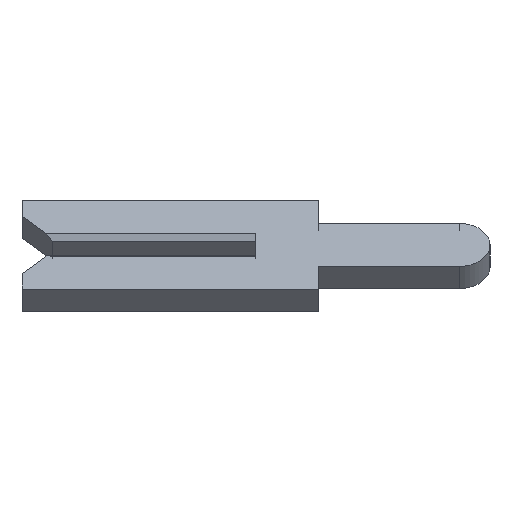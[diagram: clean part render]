
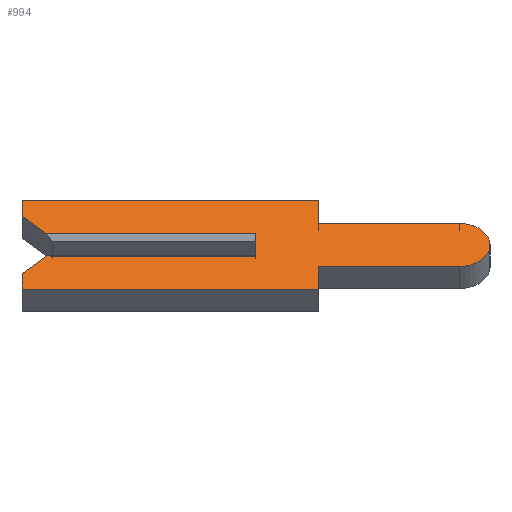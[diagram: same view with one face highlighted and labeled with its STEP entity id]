
A CAD part, left-side view. The second image highlights one B-rep face of the part: STEP entity #994.
In plain terms, the highlighted face is planar.
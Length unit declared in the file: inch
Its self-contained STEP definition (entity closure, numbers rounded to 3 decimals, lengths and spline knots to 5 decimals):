
#24 = VECTOR ( 'NONE', #486, 39.37008 ) ;
#33 = CARTESIAN_POINT ( 'NONE',  ( -0.01, -0.04, -0.04 ) ) ;
#35 = VERTEX_POINT ( 'NONE', #1326 ) ;
#36 = CARTESIAN_POINT ( 'NONE',  ( -0.01, 0.1305, -0.0065 ) ) ;
#39 = DIRECTION ( 'NONE',  ( 0., -0.707, 0.707 ) ) ;
#102 = EDGE_CURVE ( 'NONE', #569, #1413, #1185, .T. ) ;
#128 = CARTESIAN_POINT ( 'NONE',  ( -0.01, -0.04, 0.0195 ) ) ;
#132 = CARTESIAN_POINT ( 'NONE',  ( -0.01, 0.15, -0.04 ) ) ;
#154 = DIRECTION ( 'NONE',  ( 0., 0.707, 0.707 ) ) ;
#156 = EDGE_CURVE ( 'NONE', #281, #1231, #1251, .T. ) ;
#157 = VERTEX_POINT ( 'NONE', #472 ) ;
#158 = CARTESIAN_POINT ( 'NONE',  ( -0.01, 0.15, 0.04 ) ) ;
#165 = LINE ( 'NONE', #128, #1533 ) ;
#169 = LINE ( 'NONE', #1474, #1319 ) ;
#188 = DIRECTION ( 'NONE',  ( 0., -1., 0. ) ) ;
#198 = PLANE ( 'NONE',  #1428 ) ;
#204 = VECTOR ( 'NONE', #347, 39.37008 ) ;
#212 = ORIENTED_EDGE ( 'NONE', *, *, #927, .T. ) ;
#229 = CARTESIAN_POINT ( 'NONE',  ( -0.01, 0., 0.0065 ) ) ;
#237 = LINE ( 'NONE', #675, #1162 ) ;
#255 = EDGE_CURVE ( 'NONE', #788, #157, #1330, .T. ) ;
#275 = DIRECTION ( 'NONE',  ( 0., 0., -1. ) ) ;
#281 = VERTEX_POINT ( 'NONE', #132 ) ;
#306 = CARTESIAN_POINT ( 'NONE',  ( -0.01, -0.04, 0.04 ) ) ;
#311 = DIRECTION ( 'NONE',  ( 0., 0., -1. ) ) ;
#315 = ORIENTED_EDGE ( 'NONE', *, *, #1003, .F. ) ;
#321 = DIRECTION ( 'NONE',  ( 1., 0., 0. ) ) ;
#339 = EDGE_CURVE ( 'NONE', #1231, #1271, #1350, .T. ) ;
#347 = DIRECTION ( 'NONE',  ( 0., 0., 1. ) ) ;
#354 = VECTOR ( 'NONE', #188, 39.37008 ) ;
#362 = ORIENTED_EDGE ( 'NONE', *, *, #102, .F. ) ;
#424 = EDGE_CURVE ( 'NONE', #673, #788, #1155, .T. ) ;
#437 = EDGE_LOOP ( 'NONE', ( #212, #362, #588, #690, #961, #549, #1166, #315, #937, #693, #1250, #1091, #747, #1484 ) ) ;
#443 = VERTEX_POINT ( 'NONE', #644 ) ;
#448 = VECTOR ( 'NONE', #963, 39.37008 ) ;
#472 = CARTESIAN_POINT ( 'NONE',  ( -0.01, -0.04, 0.0195 ) ) ;
#486 = DIRECTION ( 'NONE',  ( 0., 0., 1. ) ) ;
#513 = CARTESIAN_POINT ( 'NONE',  ( -0.01, -0.04, 0.04 ) ) ;
#524 = VECTOR ( 'NONE', #1315, 39.37008 ) ;
#549 = ORIENTED_EDGE ( 'NONE', *, *, #1340, .F. ) ;
#564 = CARTESIAN_POINT ( 'NONE',  ( -0.01, 0.15, 0.01 ) ) ;
#569 = VERTEX_POINT ( 'NONE', #1365 ) ;
#574 = VECTOR ( 'NONE', #275, 39.37008 ) ;
#588 = ORIENTED_EDGE ( 'NONE', *, *, #1308, .F. ) ;
#644 = CARTESIAN_POINT ( 'NONE',  ( -0.01, -0.1305, 0.0195 ) ) ;
#670 = DIRECTION ( 'NONE',  ( 0., 0., -1. ) ) ;
#673 = VERTEX_POINT ( 'NONE', #158 ) ;
#674 = VERTEX_POINT ( 'NONE', #1497 ) ;
#675 = CARTESIAN_POINT ( 'NONE',  ( -0.01, -0.04, -0.0195 ) ) ;
#690 = ORIENTED_EDGE ( 'NONE', *, *, #339, .F. ) ;
#693 = ORIENTED_EDGE ( 'NONE', *, *, #1163, .F. ) ;
#703 = LINE ( 'NONE', #704, #204 ) ;
#704 = CARTESIAN_POINT ( 'NONE',  ( -0.01, 0.15, 0.026 ) ) ;
#711 = CARTESIAN_POINT ( 'NONE',  ( -0.01, 0.134, -0.01 ) ) ;
#715 = VECTOR ( 'NONE', #39, 39.37008 ) ;
#747 = ORIENTED_EDGE ( 'NONE', *, *, #1143, .F. ) ;
#756 = LINE ( 'NONE', #1197, #448 ) ;
#788 = VERTEX_POINT ( 'NONE', #306 ) ;
#820 = CARTESIAN_POINT ( 'NONE',  ( -0.01, -0.04, -0.04 ) ) ;
#890 = CARTESIAN_POINT ( 'NONE',  ( -0.01, 0.15, 0.04 ) ) ;
#905 = CARTESIAN_POINT ( 'NONE',  ( -0.01, -0.1305, 0. ) ) ;
#916 = CIRCLE ( 'NONE', #932, 0.0195 ) ;
#927 = EDGE_CURVE ( 'NONE', #35, #1413, #1416, .T. ) ;
#932 = AXIS2_PLACEMENT_3D ( 'NONE', #905, #1017, #311 ) ;
#937 = ORIENTED_EDGE ( 'NONE', *, *, #1055, .F. ) ;
#949 = CARTESIAN_POINT ( 'NONE',  ( -0.01, 0.15, -0.026 ) ) ;
#961 = ORIENTED_EDGE ( 'NONE', *, *, #156, .F. ) ;
#963 = DIRECTION ( 'NONE',  ( 0., -1., 0. ) ) ;
#972 = DIRECTION ( 'NONE',  ( 0., 0., -1. ) ) ;
#994 = ADVANCED_FACE ( 'NONE', ( #1159 ), #198, .F. ) ;
#1003 = EDGE_CURVE ( 'NONE', #674, #1069, #237, .T. ) ;
#1017 = DIRECTION ( 'NONE',  ( 1., 0., 0. ) ) ;
#1032 = VERTEX_POINT ( 'NONE', #1394 ) ;
#1044 = VECTOR ( 'NONE', #972, 39.37008 ) ;
#1046 = LINE ( 'NONE', #33, #1044 ) ;
#1055 = EDGE_CURVE ( 'NONE', #443, #674, #916, .T. ) ;
#1063 = DIRECTION ( 'NONE',  ( 0., 0., 1. ) ) ;
#1069 = VERTEX_POINT ( 'NONE', #1401 ) ;
#1091 = ORIENTED_EDGE ( 'NONE', *, *, #424, .F. ) ;
#1138 = DIRECTION ( 'NONE',  ( 0., 1., 0. ) ) ;
#1143 = EDGE_CURVE ( 'NONE', #1032, #673, #703, .T. ) ;
#1151 = CARTESIAN_POINT ( 'NONE',  ( -0.01, -0.1305, 0. ) ) ;
#1155 = LINE ( 'NONE', #890, #1391 ) ;
#1159 = FACE_OUTER_BOUND ( 'NONE', #437, .T. ) ;
#1162 = VECTOR ( 'NONE', #1138, 39.37008 ) ;
#1163 = EDGE_CURVE ( 'NONE', #157, #443, #165, .T. ) ;
#1166 = ORIENTED_EDGE ( 'NONE', *, *, #1511, .F. ) ;
#1185 = LINE ( 'NONE', #229, #1485 ) ;
#1187 = VERTEX_POINT ( 'NONE', #820 ) ;
#1189 = DIRECTION ( 'NONE',  ( 0., -1., 0. ) ) ;
#1197 = CARTESIAN_POINT ( 'NONE',  ( -0.01, -0.1305, -0.01 ) ) ;
#1231 = VERTEX_POINT ( 'NONE', #1437 ) ;
#1250 = ORIENTED_EDGE ( 'NONE', *, *, #255, .F. ) ;
#1251 = LINE ( 'NONE', #949, #24 ) ;
#1271 = VERTEX_POINT ( 'NONE', #711 ) ;
#1308 = EDGE_CURVE ( 'NONE', #1271, #569, #756, .T. ) ;
#1315 = DIRECTION ( 'NONE',  ( 0., 1., 0. ) ) ;
#1319 = VECTOR ( 'NONE', #154, 39.37008 ) ;
#1323 = CARTESIAN_POINT ( 'NONE',  ( -0.01, 0.15, -0.04 ) ) ;
#1326 = CARTESIAN_POINT ( 'NONE',  ( -0.01, 0.134, 0.01 ) ) ;
#1330 = LINE ( 'NONE', #513, #574 ) ;
#1340 = EDGE_CURVE ( 'NONE', #1187, #281, #1495, .T. ) ;
#1350 = LINE ( 'NONE', #36, #715 ) ;
#1365 = CARTESIAN_POINT ( 'NONE',  ( -0.01, 0., -0.01 ) ) ;
#1371 = DIRECTION ( 'NONE',  ( 0., -1., 0. ) ) ;
#1391 = VECTOR ( 'NONE', #1371, 39.37008 ) ;
#1394 = CARTESIAN_POINT ( 'NONE',  ( -0.01, 0.15, 0.026 ) ) ;
#1401 = CARTESIAN_POINT ( 'NONE',  ( -0.01, -0.04, -0.0195 ) ) ;
#1413 = VERTEX_POINT ( 'NONE', #1463 ) ;
#1416 = LINE ( 'NONE', #564, #354 ) ;
#1428 = AXIS2_PLACEMENT_3D ( 'NONE', #1151, #321, #670 ) ;
#1437 = CARTESIAN_POINT ( 'NONE',  ( -0.01, 0.15, -0.026 ) ) ;
#1463 = CARTESIAN_POINT ( 'NONE',  ( -0.01, 0., 0.01 ) ) ;
#1474 = CARTESIAN_POINT ( 'NONE',  ( -0.01, 0.1305, 0.0065 ) ) ;
#1484 = ORIENTED_EDGE ( 'NONE', *, *, #1534, .F. ) ;
#1485 = VECTOR ( 'NONE', #1063, 39.37008 ) ;
#1495 = LINE ( 'NONE', #1323, #524 ) ;
#1497 = CARTESIAN_POINT ( 'NONE',  ( -0.01, -0.1305, -0.0195 ) ) ;
#1511 = EDGE_CURVE ( 'NONE', #1069, #1187, #1046, .T. ) ;
#1533 = VECTOR ( 'NONE', #1189, 39.37008 ) ;
#1534 = EDGE_CURVE ( 'NONE', #35, #1032, #169, .T. ) ;
